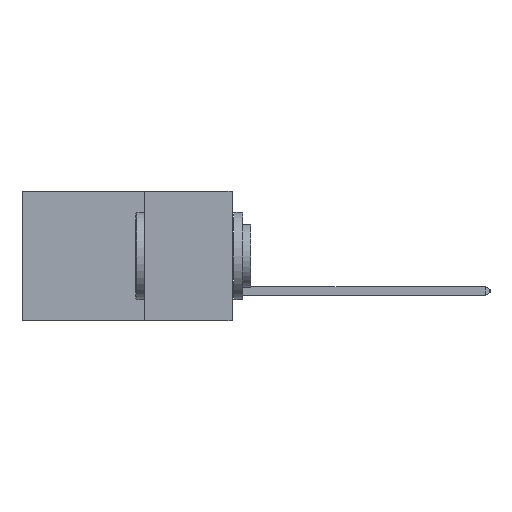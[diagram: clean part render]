
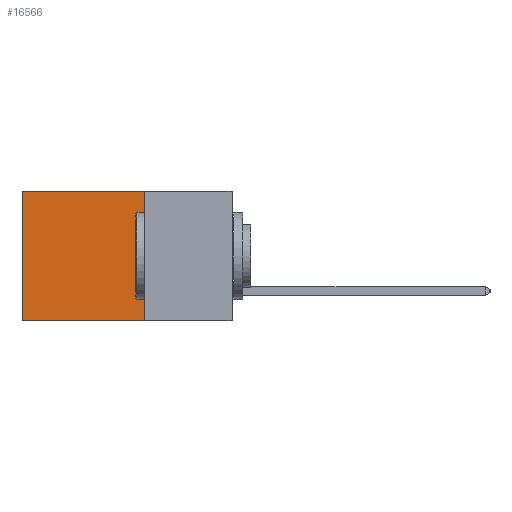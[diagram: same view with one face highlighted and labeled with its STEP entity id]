
A CAD part, left-side view. The second image highlights one B-rep face of the part: STEP entity #16566.
In plain terms, the highlighted planar face has unit normal (-1, 0, 0).
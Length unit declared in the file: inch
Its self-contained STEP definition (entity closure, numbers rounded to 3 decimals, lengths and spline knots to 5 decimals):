
#132 = DIRECTION ( 'NONE',  ( 0., 0., -1. ) ) ;
#671 = ORIENTED_EDGE ( 'NONE', *, *, #2024, .T. ) ;
#1273 = CARTESIAN_POINT ( 'NONE',  ( 0.2875, 0.25, 0. ) ) ;
#1950 = CARTESIAN_POINT ( 'NONE',  ( 0.2875, 0.6, 0. ) ) ;
#2024 = EDGE_CURVE ( 'NONE', #12436, #20900, #8396, .T. ) ;
#2930 = VERTEX_POINT ( 'NONE', #14078 ) ;
#3068 = LINE ( 'NONE', #1273, #21741 ) ;
#3151 = ORIENTED_EDGE ( 'NONE', *, *, #17784, .F. ) ;
#4175 = PLANE ( 'NONE',  #11209 ) ;
#4996 = ORIENTED_EDGE ( 'NONE', *, *, #16621, .F. ) ;
#5041 = VECTOR ( 'NONE', #5390, 39.37008 ) ;
#5390 = DIRECTION ( 'NONE',  ( 0., 0., -1. ) ) ;
#5726 = ORIENTED_EDGE ( 'NONE', *, *, #9460, .T. ) ;
#5990 = DIRECTION ( 'NONE',  ( 1., 0., 0. ) ) ;
#6140 = DIRECTION ( 'NONE',  ( 0., 1., 0. ) ) ;
#7061 = VECTOR ( 'NONE', #6140, 39.37008 ) ;
#7831 = VECTOR ( 'NONE', #132, 39.37008 ) ;
#8092 = EDGE_LOOP ( 'NONE', ( #671, #4996, #3151, #5726 ) ) ;
#8396 = LINE ( 'NONE', #1950, #7831 ) ;
#9460 = EDGE_CURVE ( 'NONE', #2930, #12436, #3068, .T. ) ;
#11209 = AXIS2_PLACEMENT_3D ( 'NONE', #16791, #5990, #18631 ) ;
#11460 = CARTESIAN_POINT ( 'NONE',  ( 0.2875, 0.6, -0.37 ) ) ;
#12436 = VERTEX_POINT ( 'NONE', #14638 ) ;
#12958 = FACE_OUTER_BOUND ( 'NONE', #8092, .T. ) ;
#13291 = CARTESIAN_POINT ( 'NONE',  ( 0.2875, 0.25, -0.37 ) ) ;
#13462 = LINE ( 'NONE', #16179, #5041 ) ;
#14056 = CARTESIAN_POINT ( 'NONE',  ( 0.2875, 0.25, -0.37 ) ) ;
#14078 = CARTESIAN_POINT ( 'NONE',  ( 0.2875, 0.25, 0. ) ) ;
#14638 = CARTESIAN_POINT ( 'NONE',  ( 0.2875, 0.6, 0. ) ) ;
#16179 = CARTESIAN_POINT ( 'NONE',  ( 0.2875, 0.25, 0. ) ) ;
#16566 = ADVANCED_FACE ( 'NONE', ( #12958 ), #4175, .F. ) ;
#16621 = EDGE_CURVE ( 'NONE', #16908, #20900, #16667, .T. ) ;
#16667 = LINE ( 'NONE', #13291, #7061 ) ;
#16791 = CARTESIAN_POINT ( 'NONE',  ( 0.2875, 0.25, 0. ) ) ;
#16908 = VERTEX_POINT ( 'NONE', #14056 ) ;
#17784 = EDGE_CURVE ( 'NONE', #2930, #16908, #13462, .T. ) ;
#18631 = DIRECTION ( 'NONE',  ( 0., 0., -1. ) ) ;
#19357 = DIRECTION ( 'NONE',  ( 0., 1., 0. ) ) ;
#20900 = VERTEX_POINT ( 'NONE', #11460 ) ;
#21741 = VECTOR ( 'NONE', #19357, 39.37008 ) ;
